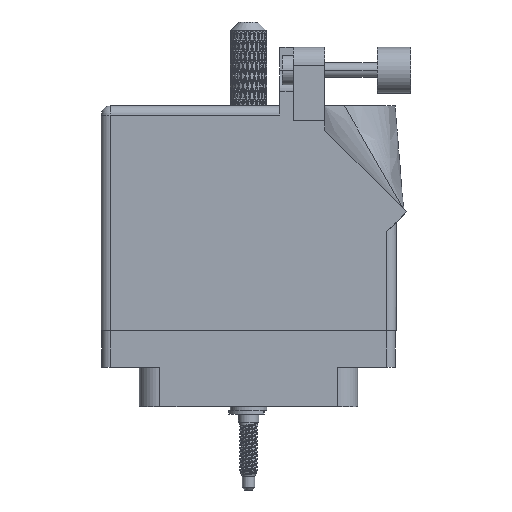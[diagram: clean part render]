
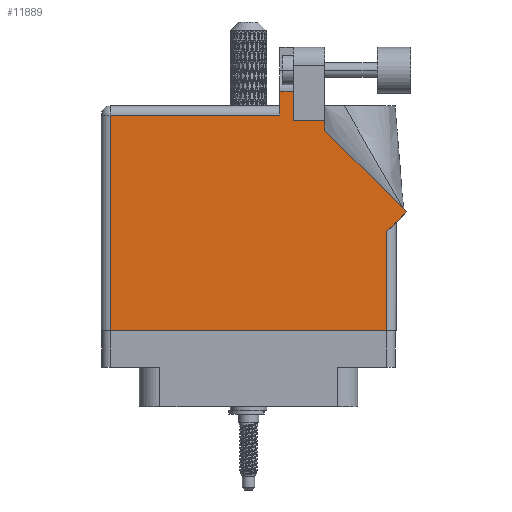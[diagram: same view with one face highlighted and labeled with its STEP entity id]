
A CAD part, front view. The second image highlights one B-rep face of the part: STEP entity #11889.
In plain terms, the highlighted face is planar.
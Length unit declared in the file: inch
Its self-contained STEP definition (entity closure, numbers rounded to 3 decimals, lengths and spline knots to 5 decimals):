
#1059 = LINE ( 'NONE', #62840, #82579 ) ;
#1591 = CARTESIAN_POINT ( 'NONE',  ( 0.212, 1.368, 0.455 ) ) ;
#1681 = VERTEX_POINT ( 'NONE', #13033 ) ;
#2224 = ORIENTED_EDGE ( 'NONE', *, *, #69294, .T. ) ;
#2656 = EDGE_CURVE ( 'NONE', #42420, #55294, #49733, .T. ) ;
#3691 = VERTEX_POINT ( 'NONE', #1591 ) ;
#6132 = VECTOR ( 'NONE', #55507, 39.37008 ) ;
#7677 = EDGE_CURVE ( 'NONE', #3691, #70012, #1059, .T. ) ;
#7793 = CARTESIAN_POINT ( 'NONE',  ( 0.306, 1.33, 0.455 ) ) ;
#8801 = EDGE_CURVE ( 'NONE', #34106, #87225, #40431, .T. ) ;
#11485 = CARTESIAN_POINT ( 'NONE',  ( 0.306, 1.5315, 0.455 ) ) ;
#11889 = ADVANCED_FACE ( 'NONE', ( #38698 ), #93022, .F. ) ;
#12953 = ORIENTED_EDGE ( 'NONE', *, *, #78003, .T. ) ;
#13033 = CARTESIAN_POINT ( 'NONE',  ( 0.519, 1.33, 0.455 ) ) ;
#13393 = EDGE_CURVE ( 'NONE', #1681, #29460, #27250, .T. ) ;
#16935 = ORIENTED_EDGE ( 'NONE', *, *, #54668, .T. ) ;
#20136 = VECTOR ( 'NONE', #44662, 39.37008 ) ;
#20883 = LINE ( 'NONE', #86893, #6132 ) ;
#21999 = VECTOR ( 'NONE', #70429, 39.37008 ) ;
#22763 = EDGE_CURVE ( 'NONE', #73230, #3691, #69551, .T. ) ;
#23004 = CARTESIAN_POINT ( 'NONE',  ( 1.07571, 0.70771, 0.455 ) ) ;
#24110 = DIRECTION ( 'NONE',  ( -1., 0., 0. ) ) ;
#24156 = DIRECTION ( 'NONE',  ( 0., 1., 0. ) ) ;
#26145 = ORIENTED_EDGE ( 'NONE', *, *, #7677, .T. ) ;
#26303 = ORIENTED_EDGE ( 'NONE', *, *, #13393, .T. ) ;
#27250 = LINE ( 'NONE', #71482, #74235 ) ;
#27730 = EDGE_CURVE ( 'NONE', #44936, #73230, #96074, .T. ) ;
#29153 = CARTESIAN_POINT ( 'NONE',  ( -1.005, 1.43, 0.455 ) ) ;
#29460 = VERTEX_POINT ( 'NONE', #7793 ) ;
#31598 = ORIENTED_EDGE ( 'NONE', *, *, #63621, .T. ) ;
#34106 = VERTEX_POINT ( 'NONE', #77343 ) ;
#35894 = ORIENTED_EDGE ( 'NONE', *, *, #2656, .T. ) ;
#37873 = CARTESIAN_POINT ( 'NONE',  ( 0.63677, 1.5315, 0.455 ) ) ;
#38698 = FACE_OUTER_BOUND ( 'NONE', #42880, .T. ) ;
#39502 = LINE ( 'NONE', #87131, #53116 ) ;
#39898 = CARTESIAN_POINT ( 'NONE',  ( 1.07571, 0.70771, 0.455 ) ) ;
#40431 = LINE ( 'NONE', #60415, #78694 ) ;
#42420 = VERTEX_POINT ( 'NONE', #72611 ) ;
#42880 = EDGE_LOOP ( 'NONE', ( #12953, #56824, #46353, #26145, #2224, #35894, #31598, #82644, #57806, #16935, #26303 ) ) ;
#44662 = DIRECTION ( 'NONE',  ( 1., 0., 0. ) ) ;
#44936 = VERTEX_POINT ( 'NONE', #11485 ) ;
#46353 = ORIENTED_EDGE ( 'NONE', *, *, #22763, .T. ) ;
#47513 = DIRECTION ( 'NONE',  ( -0.707, 0.707, 0. ) ) ;
#49733 = LINE ( 'NONE', #76457, #20136 ) ;
#51271 = CARTESIAN_POINT ( 'NONE',  ( 0.519, 1.26442, 0.455 ) ) ;
#51522 = CARTESIAN_POINT ( 'NONE',  ( 0.519, 1.26442, 0.455 ) ) ;
#53116 = VECTOR ( 'NONE', #78521, 39.37008 ) ;
#53229 = VECTOR ( 'NONE', #24156, 39.37008 ) ;
#54668 = EDGE_CURVE ( 'NONE', #71745, #1681, #79677, .T. ) ;
#55294 = VERTEX_POINT ( 'NONE', #90450 ) ;
#55507 = DIRECTION ( 'NONE',  ( 0., -1., 0. ) ) ;
#55622 = CARTESIAN_POINT ( 'NONE',  ( 0.306, 1.33, 0.455 ) ) ;
#56824 = ORIENTED_EDGE ( 'NONE', *, *, #27730, .T. ) ;
#57806 = ORIENTED_EDGE ( 'NONE', *, *, #77233, .T. ) ;
#60415 = CARTESIAN_POINT ( 'NONE',  ( 1.005, 0.637, 0.455 ) ) ;
#62840 = CARTESIAN_POINT ( 'NONE',  ( -1.005, 1.368, 0.455 ) ) ;
#63365 = AXIS2_PLACEMENT_3D ( 'NONE', #29153, #69303, #84431 ) ;
#63621 = EDGE_CURVE ( 'NONE', #55294, #34106, #39502, .T. ) ;
#65682 = LINE ( 'NONE', #23004, #80481 ) ;
#68778 = CARTESIAN_POINT ( 'NONE',  ( -0.943, 1.368, 0.455 ) ) ;
#69294 = EDGE_CURVE ( 'NONE', #70012, #42420, #20883, .T. ) ;
#69303 = DIRECTION ( 'NONE',  ( 0., 0., -1. ) ) ;
#69551 = LINE ( 'NONE', #83240, #78105 ) ;
#70012 = VERTEX_POINT ( 'NONE', #68778 ) ;
#70429 = DIRECTION ( 'NONE',  ( -1., 0., 0. ) ) ;
#71482 = CARTESIAN_POINT ( 'NONE',  ( 0.519, 1.33, 0.455 ) ) ;
#71745 = VERTEX_POINT ( 'NONE', #51522 ) ;
#72611 = CARTESIAN_POINT ( 'NONE',  ( -0.943, -0.1, 0.455 ) ) ;
#73230 = VERTEX_POINT ( 'NONE', #96669 ) ;
#74092 = DIRECTION ( 'NONE',  ( 0., 1., 0. ) ) ;
#74235 = VECTOR ( 'NONE', #24110, 39.37008 ) ;
#76457 = CARTESIAN_POINT ( 'NONE',  ( -1.005, -0.1, 0.455 ) ) ;
#77233 = EDGE_CURVE ( 'NONE', #87225, #71745, #65682, .T. ) ;
#77343 = CARTESIAN_POINT ( 'NONE',  ( 0.943, 0.575, 0.455 ) ) ;
#78003 = EDGE_CURVE ( 'NONE', #29460, #44936, #101335, .T. ) ;
#78105 = VECTOR ( 'NONE', #83922, 39.37008 ) ;
#78521 = DIRECTION ( 'NONE',  ( 0., 1., 0. ) ) ;
#78694 = VECTOR ( 'NONE', #83520, 39.37008 ) ;
#79677 = LINE ( 'NONE', #51271, #93220 ) ;
#79692 = DIRECTION ( 'NONE',  ( -1., 0., 0. ) ) ;
#80481 = VECTOR ( 'NONE', #47513, 39.37008 ) ;
#82579 = VECTOR ( 'NONE', #79692, 39.37008 ) ;
#82644 = ORIENTED_EDGE ( 'NONE', *, *, #8801, .T. ) ;
#83240 = CARTESIAN_POINT ( 'NONE',  ( 0.212, 1.43, 0.455 ) ) ;
#83520 = DIRECTION ( 'NONE',  ( 0.707, 0.707, 0. ) ) ;
#83922 = DIRECTION ( 'NONE',  ( 0., -1., 0. ) ) ;
#84431 = DIRECTION ( 'NONE',  ( -1., 0., 0. ) ) ;
#86893 = CARTESIAN_POINT ( 'NONE',  ( -0.943, -0.1, 0.455 ) ) ;
#87131 = CARTESIAN_POINT ( 'NONE',  ( 0.943, 0.637, 0.455 ) ) ;
#87225 = VERTEX_POINT ( 'NONE', #39898 ) ;
#90450 = CARTESIAN_POINT ( 'NONE',  ( 0.943, -0.1, 0.455 ) ) ;
#93022 = PLANE ( 'NONE',  #63365 ) ;
#93220 = VECTOR ( 'NONE', #74092, 39.37008 ) ;
#96074 = LINE ( 'NONE', #37873, #21999 ) ;
#96669 = CARTESIAN_POINT ( 'NONE',  ( 0.212, 1.5315, 0.455 ) ) ;
#101335 = LINE ( 'NONE', #55622, #53229 ) ;
